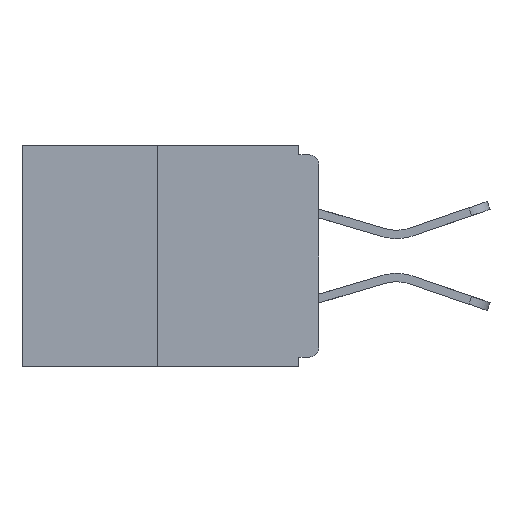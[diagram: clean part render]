
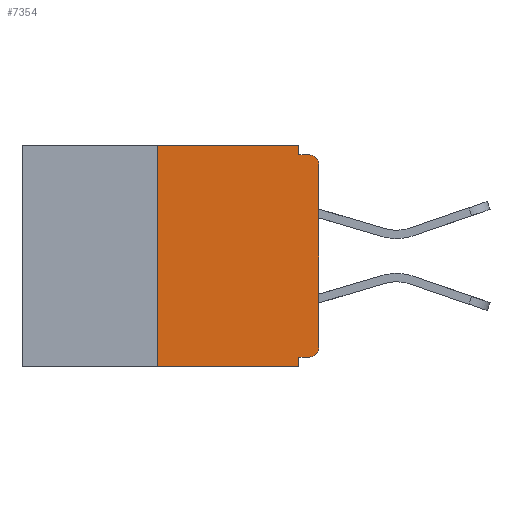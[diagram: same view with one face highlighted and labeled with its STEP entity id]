
A CAD part, left-side view. The second image highlights one B-rep face of the part: STEP entity #7354.
In plain terms, the highlighted planar face has unit normal (-1, 0, 0).
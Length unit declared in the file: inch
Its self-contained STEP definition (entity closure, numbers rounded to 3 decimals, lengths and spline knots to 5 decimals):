
#96 = ORIENTED_EDGE ( 'NONE', *, *, #7298, .F. ) ;
#115 = DIRECTION ( 'NONE',  ( 0., 0., 1. ) ) ;
#629 = DIRECTION ( 'NONE',  ( 0., 0., -1. ) ) ;
#1053 = VECTOR ( 'NONE', #1774, 39.37008 ) ;
#1352 = VECTOR ( 'NONE', #629, 39.37008 ) ;
#1696 = CARTESIAN_POINT ( 'NONE',  ( 0., 0., -0.328 ) ) ;
#1774 = DIRECTION ( 'NONE',  ( 0., 1., 0. ) ) ;
#1974 = DIRECTION ( 'NONE',  ( 0., 0., -1. ) ) ;
#2003 = DIRECTION ( 'NONE',  ( 0., 0., -1. ) ) ;
#2459 = CARTESIAN_POINT ( 'NONE',  ( 0., 0.031, -0.328 ) ) ;
#2707 = FACE_OUTER_BOUND ( 'NONE', #9040, .T. ) ;
#3033 = CARTESIAN_POINT ( 'NONE',  ( 0., 0., -0.313 ) ) ;
#3175 = DIRECTION ( 'NONE',  ( -1., 0., 0. ) ) ;
#3322 = ORIENTED_EDGE ( 'NONE', *, *, #10853, .F. ) ;
#3891 = LINE ( 'NONE', #11096, #5592 ) ;
#3921 = CARTESIAN_POINT ( 'NONE',  ( 0., 0.015, -0.015 ) ) ;
#3952 = EDGE_CURVE ( 'NONE', #5626, #14225, #13342, .T. ) ;
#4462 = ORIENTED_EDGE ( 'NONE', *, *, #14023, .T. ) ;
#4689 = VECTOR ( 'NONE', #14489, 39.37008 ) ;
#4840 = VERTEX_POINT ( 'NONE', #2459 ) ;
#4995 = CARTESIAN_POINT ( 'NONE',  ( 0., 0.031, 0. ) ) ;
#5063 = CARTESIAN_POINT ( 'NONE',  ( 0., 0.25, 0. ) ) ;
#5167 = VERTEX_POINT ( 'NONE', #9391 ) ;
#5592 = VECTOR ( 'NONE', #8515, 39.37008 ) ;
#5626 = VERTEX_POINT ( 'NONE', #5063 ) ;
#5684 = ORIENTED_EDGE ( 'NONE', *, *, #9520, .T. ) ;
#5833 = VERTEX_POINT ( 'NONE', #14390 ) ;
#5907 = CIRCLE ( 'NONE', #9221, 0.015 ) ;
#6096 = CARTESIAN_POINT ( 'NONE',  ( 0., 0.25, 0. ) ) ;
#6160 = VECTOR ( 'NONE', #13859, 39.37008 ) ;
#6232 = DIRECTION ( 'NONE',  ( 0., -1., 0. ) ) ;
#6319 = CARTESIAN_POINT ( 'NONE',  ( 0., 0.46, 0. ) ) ;
#6339 = LINE ( 'NONE', #6096, #10240 ) ;
#6697 = CARTESIAN_POINT ( 'NONE',  ( 0., 0.015, -0.313 ) ) ;
#6822 = VERTEX_POINT ( 'NONE', #7331 ) ;
#6986 = ORIENTED_EDGE ( 'NONE', *, *, #13456, .F. ) ;
#7298 = EDGE_CURVE ( 'NONE', #4840, #14028, #11415, .T. ) ;
#7331 = CARTESIAN_POINT ( 'NONE',  ( 0., 0.031, -0.015 ) ) ;
#7354 = ADVANCED_FACE ( 'NONE', ( #2707 ), #7573, .F. ) ;
#7380 = CIRCLE ( 'NONE', #9672, 0.015 ) ;
#7445 = VECTOR ( 'NONE', #7692, 39.37008 ) ;
#7573 = PLANE ( 'NONE',  #8204 ) ;
#7575 = ORIENTED_EDGE ( 'NONE', *, *, #3952, .F. ) ;
#7628 = ORIENTED_EDGE ( 'NONE', *, *, #11886, .T. ) ;
#7692 = DIRECTION ( 'NONE',  ( 0., 0., 1. ) ) ;
#8042 = ORIENTED_EDGE ( 'NONE', *, *, #9757, .F. ) ;
#8204 = AXIS2_PLACEMENT_3D ( 'NONE', #10203, #12437, #15063 ) ;
#8515 = DIRECTION ( 'NONE',  ( 0., -1., 0. ) ) ;
#9040 = EDGE_LOOP ( 'NONE', ( #7575, #14088, #4462, #96, #3322, #5684, #11791, #7628, #8042, #6986 ) ) ;
#9070 = CARTESIAN_POINT ( 'NONE',  ( 0., 0.015, -0.03 ) ) ;
#9213 = LINE ( 'NONE', #15192, #7445 ) ;
#9221 = AXIS2_PLACEMENT_3D ( 'NONE', #9070, #3175, #1974 ) ;
#9266 = VERTEX_POINT ( 'NONE', #3033 ) ;
#9391 = CARTESIAN_POINT ( 'NONE',  ( 0., 0.015, -0.328 ) ) ;
#9520 = EDGE_CURVE ( 'NONE', #5167, #9266, #7380, .T. ) ;
#9672 = AXIS2_PLACEMENT_3D ( 'NONE', #6697, #10220, #2003 ) ;
#9757 = EDGE_CURVE ( 'NONE', #6822, #14574, #3891, .T. ) ;
#10203 = CARTESIAN_POINT ( 'NONE',  ( 0., 0.46, 0. ) ) ;
#10220 = DIRECTION ( 'NONE',  ( -1., 0., 0. ) ) ;
#10240 = VECTOR ( 'NONE', #115, 39.37008 ) ;
#10370 = CARTESIAN_POINT ( 'NONE',  ( 0., 0.031, -0.343 ) ) ;
#10688 = CARTESIAN_POINT ( 'NONE',  ( 0., 0.46, -0.343 ) ) ;
#10853 = EDGE_CURVE ( 'NONE', #5167, #4840, #12631, .T. ) ;
#11096 = CARTESIAN_POINT ( 'NONE',  ( 0., 0., -0.015 ) ) ;
#11415 = LINE ( 'NONE', #10370, #6160 ) ;
#11473 = VERTEX_POINT ( 'NONE', #13310 ) ;
#11527 = VECTOR ( 'NONE', #6232, 39.37008 ) ;
#11791 = ORIENTED_EDGE ( 'NONE', *, *, #12235, .T. ) ;
#11886 = EDGE_CURVE ( 'NONE', #5833, #14574, #5907, .T. ) ;
#12053 = EDGE_CURVE ( 'NONE', #11473, #5626, #6339, .T. ) ;
#12235 = EDGE_CURVE ( 'NONE', #9266, #5833, #9213, .T. ) ;
#12437 = DIRECTION ( 'NONE',  ( 1., 0., 0. ) ) ;
#12631 = LINE ( 'NONE', #1696, #1053 ) ;
#13149 = LINE ( 'NONE', #10688, #4689 ) ;
#13310 = CARTESIAN_POINT ( 'NONE',  ( 0., 0.25, -0.343 ) ) ;
#13342 = LINE ( 'NONE', #6319, #11527 ) ;
#13456 = EDGE_CURVE ( 'NONE', #14225, #6822, #14034, .T. ) ;
#13859 = DIRECTION ( 'NONE',  ( 0., 0., -1. ) ) ;
#14023 = EDGE_CURVE ( 'NONE', #11473, #14028, #13149, .T. ) ;
#14028 = VERTEX_POINT ( 'NONE', #14333 ) ;
#14034 = LINE ( 'NONE', #15321, #1352 ) ;
#14088 = ORIENTED_EDGE ( 'NONE', *, *, #12053, .F. ) ;
#14225 = VERTEX_POINT ( 'NONE', #4995 ) ;
#14333 = CARTESIAN_POINT ( 'NONE',  ( 0., 0.031, -0.343 ) ) ;
#14390 = CARTESIAN_POINT ( 'NONE',  ( 0., 0., -0.03 ) ) ;
#14489 = DIRECTION ( 'NONE',  ( 0., -1., 0. ) ) ;
#14574 = VERTEX_POINT ( 'NONE', #3921 ) ;
#15063 = DIRECTION ( 'NONE',  ( 0., 0., -1. ) ) ;
#15192 = CARTESIAN_POINT ( 'NONE',  ( 0., 0., 0. ) ) ;
#15321 = CARTESIAN_POINT ( 'NONE',  ( 0., 0.031, 0. ) ) ;
